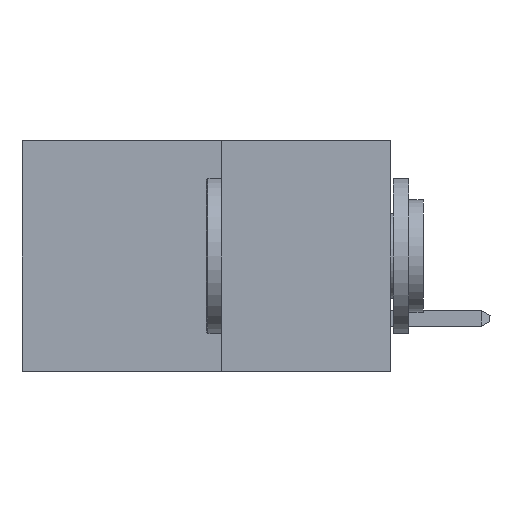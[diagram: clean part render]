
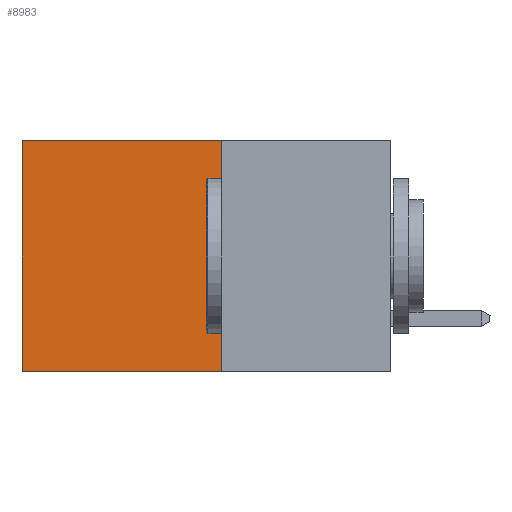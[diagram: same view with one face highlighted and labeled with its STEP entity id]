
A CAD part, left-side view. The second image highlights one B-rep face of the part: STEP entity #8983.
In plain terms, the highlighted planar face has unit normal (-1, 0, 0).
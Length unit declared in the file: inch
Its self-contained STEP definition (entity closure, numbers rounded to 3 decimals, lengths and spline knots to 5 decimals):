
#12 = DIRECTION ( 'NONE',  ( 0., 0., -1. ) ) ;
#19 = EDGE_CURVE ( 'NONE', #10524, #3038, #1957, .T. ) ;
#457 = ORIENTED_EDGE ( 'NONE', *, *, #2859, .F. ) ;
#1157 = DIRECTION ( 'NONE',  ( 0., 0., -1. ) ) ;
#1209 = LINE ( 'NONE', #10593, #8694 ) ;
#1957 = LINE ( 'NONE', #8542, #12365 ) ;
#2605 = DIRECTION ( 'NONE',  ( 0., 1., 0. ) ) ;
#2791 = VECTOR ( 'NONE', #2605, 39.37008 ) ;
#2859 = EDGE_CURVE ( 'NONE', #3038, #12253, #5738, .T. ) ;
#3038 = VERTEX_POINT ( 'NONE', #6327 ) ;
#3124 = EDGE_LOOP ( 'NONE', ( #8265, #457, #3580, #9827 ) ) ;
#3251 = EDGE_CURVE ( 'NONE', #10524, #7682, #11392, .T. ) ;
#3580 = ORIENTED_EDGE ( 'NONE', *, *, #19, .F. ) ;
#4191 = AXIS2_PLACEMENT_3D ( 'NONE', #12153, #6131, #12 ) ;
#5558 = CARTESIAN_POINT ( 'NONE',  ( 0.277, 0.59, 0. ) ) ;
#5738 = LINE ( 'NONE', #8229, #2791 ) ;
#6064 = EDGE_CURVE ( 'NONE', #7682, #12253, #1209, .T. ) ;
#6131 = DIRECTION ( 'NONE',  ( 1., 0., 0. ) ) ;
#6327 = CARTESIAN_POINT ( 'NONE',  ( 0.277, 0.27, -0.37 ) ) ;
#7682 = VERTEX_POINT ( 'NONE', #5558 ) ;
#8119 = PLANE ( 'NONE',  #4191 ) ;
#8229 = CARTESIAN_POINT ( 'NONE',  ( 0.277, 0.27, -0.37 ) ) ;
#8265 = ORIENTED_EDGE ( 'NONE', *, *, #6064, .T. ) ;
#8542 = CARTESIAN_POINT ( 'NONE',  ( 0.277, 0.27, -0.37 ) ) ;
#8694 = VECTOR ( 'NONE', #10582, 39.37008 ) ;
#8983 = ADVANCED_FACE ( 'NONE', ( #11816 ), #8119, .F. ) ;
#9172 = CARTESIAN_POINT ( 'NONE',  ( 0.277, 0.27, 0. ) ) ;
#9827 = ORIENTED_EDGE ( 'NONE', *, *, #3251, .T. ) ;
#9841 = CARTESIAN_POINT ( 'NONE',  ( 0.277, 0.27, 0. ) ) ;
#9885 = DIRECTION ( 'NONE',  ( 0., 1., 0. ) ) ;
#10524 = VERTEX_POINT ( 'NONE', #9841 ) ;
#10582 = DIRECTION ( 'NONE',  ( 0., 0., -1. ) ) ;
#10593 = CARTESIAN_POINT ( 'NONE',  ( 0.277, 0.59, -0.37 ) ) ;
#11078 = VECTOR ( 'NONE', #9885, 39.37008 ) ;
#11392 = LINE ( 'NONE', #9172, #11078 ) ;
#11816 = FACE_OUTER_BOUND ( 'NONE', #3124, .T. ) ;
#12153 = CARTESIAN_POINT ( 'NONE',  ( 0.277, 0.27, -0.37 ) ) ;
#12253 = VERTEX_POINT ( 'NONE', #12666 ) ;
#12365 = VECTOR ( 'NONE', #1157, 39.37008 ) ;
#12666 = CARTESIAN_POINT ( 'NONE',  ( 0.277, 0.59, -0.37 ) ) ;
